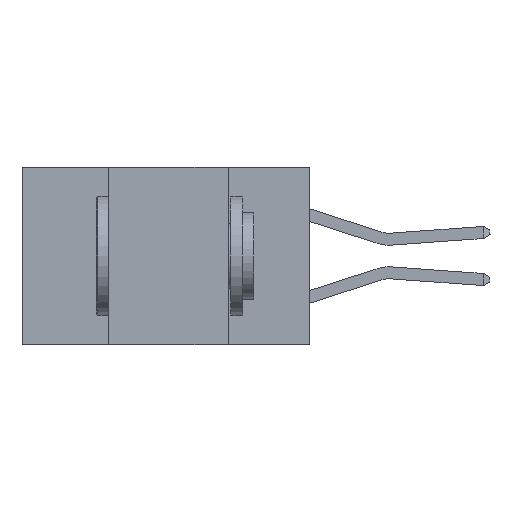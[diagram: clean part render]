
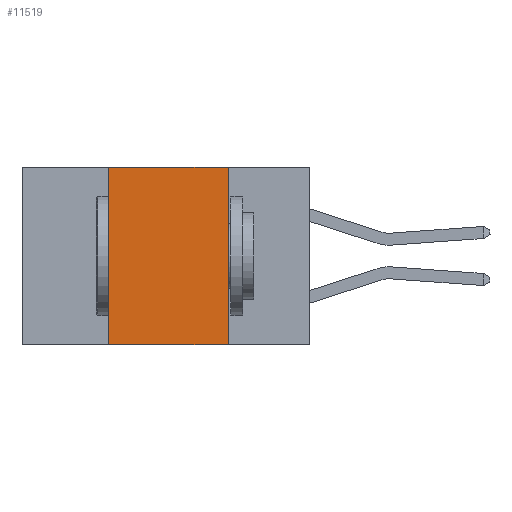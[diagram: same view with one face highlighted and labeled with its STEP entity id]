
A CAD part, left-side view. The second image highlights one B-rep face of the part: STEP entity #11519.
In plain terms, the highlighted planar face has unit normal (-1, 0, 0).
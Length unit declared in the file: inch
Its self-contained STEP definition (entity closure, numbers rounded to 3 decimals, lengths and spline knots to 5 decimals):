
#436 = CARTESIAN_POINT ( 'NONE',  ( 0., 0.17, -0.37 ) ) ;
#654 = VECTOR ( 'NONE', #5032, 39.37008 ) ;
#741 = CARTESIAN_POINT ( 'NONE',  ( 0., 0.42, -0.37 ) ) ;
#901 = CARTESIAN_POINT ( 'NONE',  ( 0., 0.17, 0. ) ) ;
#1283 = DIRECTION ( 'NONE',  ( 0., -1., 0. ) ) ;
#1973 = DIRECTION ( 'NONE',  ( 0., 0., -1. ) ) ;
#2814 = EDGE_CURVE ( 'NONE', #11261, #16214, #17619, .T. ) ;
#3460 = ORIENTED_EDGE ( 'NONE', *, *, #14072, .F. ) ;
#4176 = CARTESIAN_POINT ( 'NONE',  ( 0., 0.17, -0.37 ) ) ;
#4510 = PLANE ( 'NONE',  #15869 ) ;
#4555 = ORIENTED_EDGE ( 'NONE', *, *, #5129, .F. ) ;
#4989 = VERTEX_POINT ( 'NONE', #436 ) ;
#5032 = DIRECTION ( 'NONE',  ( 0., 0., 1. ) ) ;
#5129 = EDGE_CURVE ( 'NONE', #16214, #23815, #8916, .T. ) ;
#6028 = LINE ( 'NONE', #4176, #21791 ) ;
#8916 = LINE ( 'NONE', #22100, #21426 ) ;
#10921 = EDGE_CURVE ( 'NONE', #11261, #4989, #15806, .T. ) ;
#11261 = VERTEX_POINT ( 'NONE', #16159 ) ;
#11519 = ADVANCED_FACE ( 'NONE', ( #12048 ), #4510, .F. ) ;
#12048 = FACE_OUTER_BOUND ( 'NONE', #16904, .T. ) ;
#14072 = EDGE_CURVE ( 'NONE', #23815, #4989, #6028, .T. ) ;
#14121 = ORIENTED_EDGE ( 'NONE', *, *, #10921, .T. ) ;
#14995 = CARTESIAN_POINT ( 'NONE',  ( 0., 0.42, 0. ) ) ;
#15806 = LINE ( 'NONE', #22822, #18964 ) ;
#15869 = AXIS2_PLACEMENT_3D ( 'NONE', #21649, #17831, #19806 ) ;
#16159 = CARTESIAN_POINT ( 'NONE',  ( 0., 0.42, -0.37 ) ) ;
#16214 = VERTEX_POINT ( 'NONE', #14995 ) ;
#16904 = EDGE_LOOP ( 'NONE', ( #3460, #4555, #20211, #14121 ) ) ;
#17619 = LINE ( 'NONE', #741, #654 ) ;
#17831 = DIRECTION ( 'NONE',  ( 1., 0., 0. ) ) ;
#18964 = VECTOR ( 'NONE', #19625, 39.37008 ) ;
#19625 = DIRECTION ( 'NONE',  ( 0., -1., 0. ) ) ;
#19806 = DIRECTION ( 'NONE',  ( 0., 0., -1. ) ) ;
#20211 = ORIENTED_EDGE ( 'NONE', *, *, #2814, .F. ) ;
#21426 = VECTOR ( 'NONE', #1283, 39.37008 ) ;
#21649 = CARTESIAN_POINT ( 'NONE',  ( 0., 0.6, 0. ) ) ;
#21791 = VECTOR ( 'NONE', #1973, 39.37008 ) ;
#22100 = CARTESIAN_POINT ( 'NONE',  ( 0., 0.6, 0. ) ) ;
#22822 = CARTESIAN_POINT ( 'NONE',  ( 0., 0.6, -0.37 ) ) ;
#23815 = VERTEX_POINT ( 'NONE', #901 ) ;
